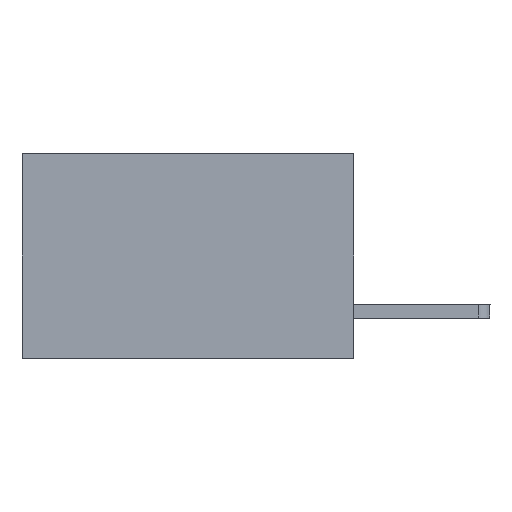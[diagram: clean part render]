
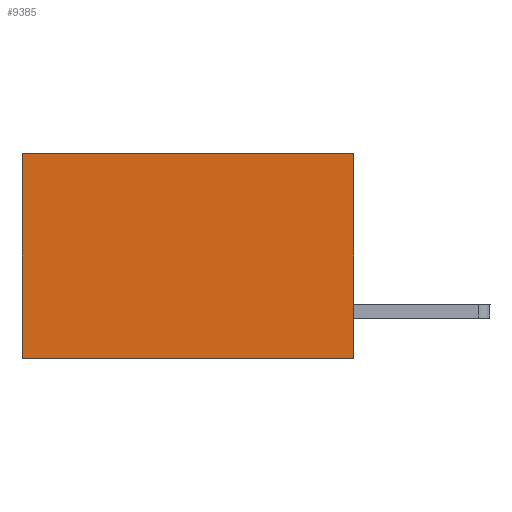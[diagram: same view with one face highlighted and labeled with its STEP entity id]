
A CAD part, left-side view. The second image highlights one B-rep face of the part: STEP entity #9385.
In plain terms, the highlighted planar face has unit normal (-1, 0, 0).
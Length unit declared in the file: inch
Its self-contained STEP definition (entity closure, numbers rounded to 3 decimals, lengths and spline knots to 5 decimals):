
#16 = CARTESIAN_POINT ( 'NONE',  ( 0.2875, 0., 0. ) ) ;
#157 = CARTESIAN_POINT ( 'NONE',  ( 0.2875, 0.6, 0. ) ) ;
#497 = CARTESIAN_POINT ( 'NONE',  ( 0.2875, 0., 0. ) ) ;
#630 = CARTESIAN_POINT ( 'NONE',  ( 0.2875, 0., -0.37 ) ) ;
#1486 = ORIENTED_EDGE ( 'NONE', *, *, #14692, .F. ) ;
#1782 = VERTEX_POINT ( 'NONE', #8255 ) ;
#2286 = VECTOR ( 'NONE', #9665, 39.37008 ) ;
#2459 = LINE ( 'NONE', #14771, #2286 ) ;
#2527 = LINE ( 'NONE', #16, #15093 ) ;
#3011 = VERTEX_POINT ( 'NONE', #630 ) ;
#5247 = DIRECTION ( 'NONE',  ( 0., 0., -1. ) ) ;
#5391 = LINE ( 'NONE', #157, #13769 ) ;
#5812 = ORIENTED_EDGE ( 'NONE', *, *, #6336, .T. ) ;
#6336 = EDGE_CURVE ( 'NONE', #1782, #13144, #2459, .T. ) ;
#7755 = DIRECTION ( 'NONE',  ( 0., 1., 0. ) ) ;
#7764 = PLANE ( 'NONE',  #11384 ) ;
#8255 = CARTESIAN_POINT ( 'NONE',  ( 0.2875, 0., 0. ) ) ;
#8654 = DIRECTION ( 'NONE',  ( 0., 0., -1. ) ) ;
#8689 = DIRECTION ( 'NONE',  ( 0., 0., -1. ) ) ;
#9047 = EDGE_CURVE ( 'NONE', #13144, #12543, #5391, .T. ) ;
#9210 = VECTOR ( 'NONE', #7755, 39.37008 ) ;
#9385 = ADVANCED_FACE ( 'NONE', ( #11083 ), #7764, .F. ) ;
#9655 = ORIENTED_EDGE ( 'NONE', *, *, #9047, .T. ) ;
#9665 = DIRECTION ( 'NONE',  ( 0., 1., 0. ) ) ;
#10709 = EDGE_LOOP ( 'NONE', ( #9655, #1486, #11420, #5812 ) ) ;
#11040 = CARTESIAN_POINT ( 'NONE',  ( 0.2875, 0.6, -0.37 ) ) ;
#11083 = FACE_OUTER_BOUND ( 'NONE', #10709, .T. ) ;
#11316 = DIRECTION ( 'NONE',  ( 1., 0., 0. ) ) ;
#11362 = CARTESIAN_POINT ( 'NONE',  ( 0.2875, 0., -0.37 ) ) ;
#11384 = AXIS2_PLACEMENT_3D ( 'NONE', #497, #11316, #5247 ) ;
#11420 = ORIENTED_EDGE ( 'NONE', *, *, #15617, .F. ) ;
#12136 = CARTESIAN_POINT ( 'NONE',  ( 0.2875, 0.6, 0. ) ) ;
#12438 = LINE ( 'NONE', #11362, #9210 ) ;
#12543 = VERTEX_POINT ( 'NONE', #11040 ) ;
#13144 = VERTEX_POINT ( 'NONE', #12136 ) ;
#13769 = VECTOR ( 'NONE', #8689, 39.37008 ) ;
#14692 = EDGE_CURVE ( 'NONE', #3011, #12543, #12438, .T. ) ;
#14771 = CARTESIAN_POINT ( 'NONE',  ( 0.2875, 0., 0. ) ) ;
#15093 = VECTOR ( 'NONE', #8654, 39.37008 ) ;
#15617 = EDGE_CURVE ( 'NONE', #1782, #3011, #2527, .T. ) ;
